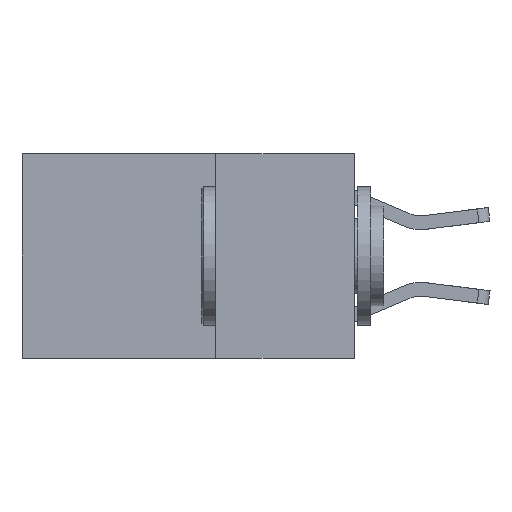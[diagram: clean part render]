
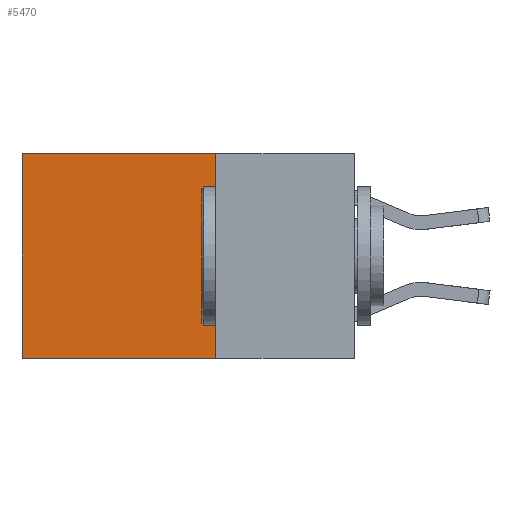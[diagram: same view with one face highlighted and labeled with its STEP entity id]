
A CAD part, left-side view. The second image highlights one B-rep face of the part: STEP entity #5470.
In plain terms, the highlighted planar face has unit normal (-1, 0, 0).
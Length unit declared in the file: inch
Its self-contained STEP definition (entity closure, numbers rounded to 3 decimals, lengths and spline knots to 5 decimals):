
#197 = DIRECTION ( 'NONE',  ( 1., 0., 0. ) ) ;
#377 = CARTESIAN_POINT ( 'NONE',  ( 0.2625, 0.25, 0. ) ) ;
#524 = LINE ( 'NONE', #5798, #8424 ) ;
#527 = CARTESIAN_POINT ( 'NONE',  ( 0.2625, 0.6, -0.37 ) ) ;
#933 = DIRECTION ( 'NONE',  ( 0., 1., 0. ) ) ;
#1195 = EDGE_CURVE ( 'NONE', #6073, #8254, #3005, .T. ) ;
#1432 = DIRECTION ( 'NONE',  ( 0., 0., -1. ) ) ;
#2134 = CARTESIAN_POINT ( 'NONE',  ( 0.2625, 0.25, -0.37 ) ) ;
#2293 = VECTOR ( 'NONE', #3069, 39.37008 ) ;
#2310 = ORIENTED_EDGE ( 'NONE', *, *, #4570, .T. ) ;
#2526 = LINE ( 'NONE', #5904, #2293 ) ;
#3005 = LINE ( 'NONE', #377, #6616 ) ;
#3069 = DIRECTION ( 'NONE',  ( 0., 1., 0. ) ) ;
#3269 = VERTEX_POINT ( 'NONE', #9080 ) ;
#3347 = EDGE_CURVE ( 'NONE', #8254, #9020, #6333, .T. ) ;
#3944 = CARTESIAN_POINT ( 'NONE',  ( 0.2625, 0.25, 0. ) ) ;
#4570 = EDGE_CURVE ( 'NONE', #3269, #9020, #524, .T. ) ;
#4575 = CARTESIAN_POINT ( 'NONE',  ( 0.2625, 0.25, 0. ) ) ;
#4842 = CARTESIAN_POINT ( 'NONE',  ( 0.2625, 0.25, -0.37 ) ) ;
#5320 = EDGE_LOOP ( 'NONE', ( #2310, #6249, #6665, #5765 ) ) ;
#5366 = DIRECTION ( 'NONE',  ( 0., 0., -1. ) ) ;
#5470 = ADVANCED_FACE ( 'NONE', ( #8539 ), #9075, .F. ) ;
#5765 = ORIENTED_EDGE ( 'NONE', *, *, #7838, .T. ) ;
#5798 = CARTESIAN_POINT ( 'NONE',  ( 0.2625, 0.6, 0. ) ) ;
#5904 = CARTESIAN_POINT ( 'NONE',  ( 0.2625, 0.25, 0. ) ) ;
#6073 = VERTEX_POINT ( 'NONE', #4575 ) ;
#6249 = ORIENTED_EDGE ( 'NONE', *, *, #3347, .F. ) ;
#6333 = LINE ( 'NONE', #2134, #6563 ) ;
#6563 = VECTOR ( 'NONE', #933, 39.37008 ) ;
#6616 = VECTOR ( 'NONE', #9054, 39.37008 ) ;
#6665 = ORIENTED_EDGE ( 'NONE', *, *, #1195, .F. ) ;
#7616 = AXIS2_PLACEMENT_3D ( 'NONE', #3944, #197, #5366 ) ;
#7838 = EDGE_CURVE ( 'NONE', #6073, #3269, #2526, .T. ) ;
#8254 = VERTEX_POINT ( 'NONE', #4842 ) ;
#8424 = VECTOR ( 'NONE', #1432, 39.37008 ) ;
#8539 = FACE_OUTER_BOUND ( 'NONE', #5320, .T. ) ;
#9020 = VERTEX_POINT ( 'NONE', #527 ) ;
#9054 = DIRECTION ( 'NONE',  ( 0., 0., -1. ) ) ;
#9075 = PLANE ( 'NONE',  #7616 ) ;
#9080 = CARTESIAN_POINT ( 'NONE',  ( 0.2625, 0.6, 0. ) ) ;
